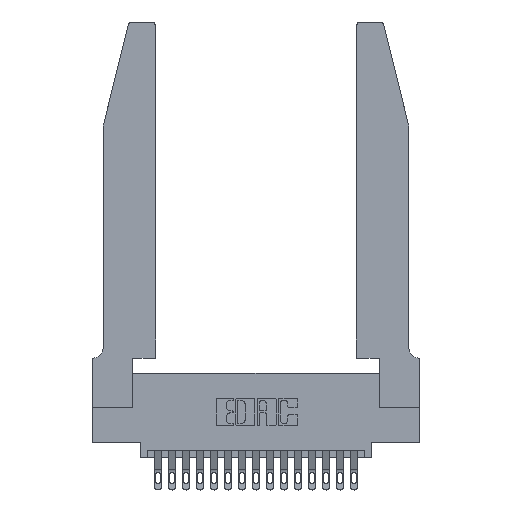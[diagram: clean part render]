
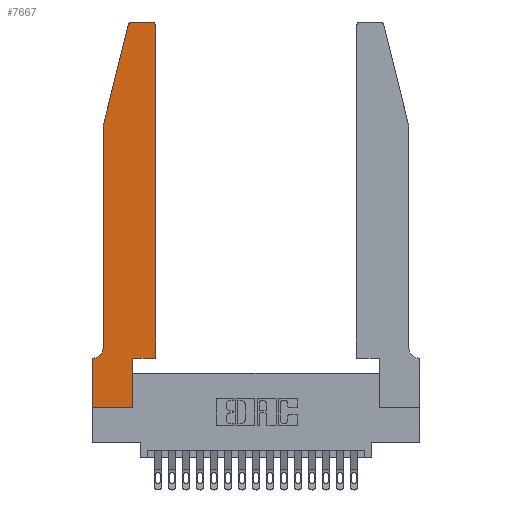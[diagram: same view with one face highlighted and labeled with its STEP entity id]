
A CAD part, top view. The second image highlights one B-rep face of the part: STEP entity #7667.
In plain terms, the highlighted planar face has unit normal (0, 0, 1).
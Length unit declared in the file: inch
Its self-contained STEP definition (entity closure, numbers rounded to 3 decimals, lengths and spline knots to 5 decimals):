
#40 = VERTEX_POINT ( 'NONE', #2530 ) ;
#57 = CARTESIAN_POINT ( 'NONE',  ( 0., 0., 0.37 ) ) ;
#232 = VERTEX_POINT ( 'NONE', #11182 ) ;
#585 = CARTESIAN_POINT ( 'NONE',  ( 0.2605, 2.75, 0.37 ) ) ;
#728 = VECTOR ( 'NONE', #1380, 39.37008 ) ;
#1380 = DIRECTION ( 'NONE',  ( 1., 0., 0. ) ) ;
#2530 = CARTESIAN_POINT ( 'NONE',  ( 0.25487, 2.72718, 0.37 ) ) ;
#2586 = VECTOR ( 'NONE', #4347, 39.37008 ) ;
#2841 = AXIS2_PLACEMENT_3D ( 'NONE', #10118, #5791, #13839 ) ;
#2979 = ORIENTED_EDGE ( 'NONE', *, *, #18411, .T. ) ;
#3191 = VERTEX_POINT ( 'NONE', #17429 ) ;
#3565 = CARTESIAN_POINT ( 'NONE',  ( 0., 0., 0.37 ) ) ;
#3614 = EDGE_CURVE ( 'NONE', #40, #8556, #8418, .T. ) ;
#3856 = AXIS2_PLACEMENT_3D ( 'NONE', #6709, #17944, #13166 ) ;
#3888 = EDGE_CURVE ( 'NONE', #16917, #5561, #12679, .T. ) ;
#4110 = ORIENTED_EDGE ( 'NONE', *, *, #10051, .T. ) ;
#4347 = DIRECTION ( 'NONE',  ( 0., -1., 0. ) ) ;
#4677 = CARTESIAN_POINT ( 'NONE',  ( 0.2865, 0., 0.37 ) ) ;
#4692 = CARTESIAN_POINT ( 'NONE',  ( 0., 0., 0.37 ) ) ;
#4755 = AXIS2_PLACEMENT_3D ( 'NONE', #7653, #12594, #9204 ) ;
#5081 = LINE ( 'NONE', #585, #10305 ) ;
#5183 = EDGE_CURVE ( 'NONE', #5561, #14321, #7615, .T. ) ;
#5474 = ORIENTED_EDGE ( 'NONE', *, *, #9919, .T. ) ;
#5485 = LINE ( 'NONE', #57, #728 ) ;
#5500 = ORIENTED_EDGE ( 'NONE', *, *, #6899, .T. ) ;
#5561 = VERTEX_POINT ( 'NONE', #11000 ) ;
#5791 = DIRECTION ( 'NONE',  ( 0., 0., 1. ) ) ;
#5873 = DIRECTION ( 'NONE',  ( 0., 0., 1. ) ) ;
#6017 = VECTOR ( 'NONE', #9428, 39.37008 ) ;
#6091 = LINE ( 'NONE', #9162, #2586 ) ;
#6281 = CIRCLE ( 'NONE', #3856, 0.03 ) ;
#6568 = EDGE_CURVE ( 'NONE', #8556, #16917, #6091, .T. ) ;
#6709 = CARTESIAN_POINT ( 'NONE',  ( 0.4205, 2.72, 0.37 ) ) ;
#6899 = EDGE_CURVE ( 'NONE', #232, #12903, #5081, .T. ) ;
#6917 = ORIENTED_EDGE ( 'NONE', *, *, #11841, .T. ) ;
#7072 = CARTESIAN_POINT ( 'NONE',  ( 0., 0.35, 0.37 ) ) ;
#7615 = LINE ( 'NONE', #15727, #12909 ) ;
#7653 = CARTESIAN_POINT ( 'NONE',  ( 0.0055, 0.42, 0.37 ) ) ;
#7667 = ADVANCED_FACE ( 'NONE', ( #14831 ), #9023, .T. ) ;
#7739 = DIRECTION ( 'NONE',  ( -1., 0., 0. ) ) ;
#7962 = EDGE_CURVE ( 'NONE', #3191, #232, #6281, .T. ) ;
#8030 = VERTEX_POINT ( 'NONE', #18083 ) ;
#8418 = LINE ( 'NONE', #9877, #16181 ) ;
#8556 = VERTEX_POINT ( 'NONE', #19950 ) ;
#8760 = ORIENTED_EDGE ( 'NONE', *, *, #9434, .T. ) ;
#8958 = CARTESIAN_POINT ( 'NONE',  ( 0.2865, 0.35, 0.37 ) ) ;
#9023 = PLANE ( 'NONE',  #11771 ) ;
#9162 = CARTESIAN_POINT ( 'NONE',  ( 0.0755, 2., 0.37 ) ) ;
#9168 = LINE ( 'NONE', #12380, #14961 ) ;
#9204 = DIRECTION ( 'NONE',  ( -1., 0., 0. ) ) ;
#9220 = DIRECTION ( 'NONE',  ( 1., 0., 0. ) ) ;
#9428 = DIRECTION ( 'NONE',  ( 0., -1., 0. ) ) ;
#9434 = EDGE_CURVE ( 'NONE', #8030, #3191, #11290, .T. ) ;
#9614 = CARTESIAN_POINT ( 'NONE',  ( 0.284, 2.75, 0.37 ) ) ;
#9857 = CARTESIAN_POINT ( 'NONE',  ( 0.2865, 0.35, 0.37 ) ) ;
#9877 = CARTESIAN_POINT ( 'NONE',  ( 0.0755, 2., 0.37 ) ) ;
#9919 = EDGE_CURVE ( 'NONE', #11551, #13581, #5485, .T. ) ;
#10051 = EDGE_CURVE ( 'NONE', #12903, #40, #12504, .T. ) ;
#10079 = DIRECTION ( 'NONE',  ( -0.239, -0.971, 0. ) ) ;
#10118 = CARTESIAN_POINT ( 'NONE',  ( 0.284, 2.72, 0.37 ) ) ;
#10142 = ORIENTED_EDGE ( 'NONE', *, *, #5183, .T. ) ;
#10295 = LINE ( 'NONE', #8958, #14060 ) ;
#10305 = VECTOR ( 'NONE', #15006, 39.37008 ) ;
#10430 = CARTESIAN_POINT ( 'NONE',  ( 0.4505, 0.35, 0.37 ) ) ;
#10916 = ORIENTED_EDGE ( 'NONE', *, *, #13179, .T. ) ;
#11000 = CARTESIAN_POINT ( 'NONE',  ( 0.0055, 0.35, 0.37 ) ) ;
#11182 = CARTESIAN_POINT ( 'NONE',  ( 0.4205, 2.75, 0.37 ) ) ;
#11290 = LINE ( 'NONE', #10430, #20212 ) ;
#11551 = VERTEX_POINT ( 'NONE', #3565 ) ;
#11652 = ORIENTED_EDGE ( 'NONE', *, *, #7962, .T. ) ;
#11771 = AXIS2_PLACEMENT_3D ( 'NONE', #18684, #5873, #20140 ) ;
#11841 = EDGE_CURVE ( 'NONE', #12798, #8030, #9168, .T. ) ;
#12380 = CARTESIAN_POINT ( 'NONE',  ( 0.4505, 0.35, 0.37 ) ) ;
#12504 = CIRCLE ( 'NONE', #2841, 0.03 ) ;
#12594 = DIRECTION ( 'NONE',  ( 0., 0., -1. ) ) ;
#12679 = CIRCLE ( 'NONE', #4755, 0.07 ) ;
#12798 = VERTEX_POINT ( 'NONE', #9857 ) ;
#12903 = VERTEX_POINT ( 'NONE', #9614 ) ;
#12909 = VECTOR ( 'NONE', #7739, 39.37008 ) ;
#13166 = DIRECTION ( 'NONE',  ( 1., 0., 0. ) ) ;
#13179 = EDGE_CURVE ( 'NONE', #13581, #12798, #10295, .T. ) ;
#13581 = VERTEX_POINT ( 'NONE', #4677 ) ;
#13839 = DIRECTION ( 'NONE',  ( 1., 0., 0. ) ) ;
#14060 = VECTOR ( 'NONE', #20078, 39.37008 ) ;
#14321 = VERTEX_POINT ( 'NONE', #7072 ) ;
#14358 = CARTESIAN_POINT ( 'NONE',  ( 0.0755, 0.42, 0.37 ) ) ;
#14831 = FACE_OUTER_BOUND ( 'NONE', #18434, .T. ) ;
#14961 = VECTOR ( 'NONE', #9220, 39.37008 ) ;
#15006 = DIRECTION ( 'NONE',  ( -1., 0., 0. ) ) ;
#15149 = DIRECTION ( 'NONE',  ( 0., 1., 0. ) ) ;
#15727 = CARTESIAN_POINT ( 'NONE',  ( 0.0755, 0.35, 0.37 ) ) ;
#16181 = VECTOR ( 'NONE', #10079, 39.37008 ) ;
#16917 = VERTEX_POINT ( 'NONE', #14358 ) ;
#17429 = CARTESIAN_POINT ( 'NONE',  ( 0.4505, 2.72, 0.37 ) ) ;
#17944 = DIRECTION ( 'NONE',  ( 0., 0., 1. ) ) ;
#18083 = CARTESIAN_POINT ( 'NONE',  ( 0.4505, 0.35, 0.37 ) ) ;
#18205 = ORIENTED_EDGE ( 'NONE', *, *, #3888, .T. ) ;
#18411 = EDGE_CURVE ( 'NONE', #14321, #11551, #19959, .T. ) ;
#18434 = EDGE_LOOP ( 'NONE', ( #5500, #4110, #20131, #20263, #18205, #10142, #2979, #5474, #10916, #6917, #8760, #11652 ) ) ;
#18684 = CARTESIAN_POINT ( 'NONE',  ( 0., 0.35, 0.37 ) ) ;
#19950 = CARTESIAN_POINT ( 'NONE',  ( 0.0755, 2., 0.37 ) ) ;
#19959 = LINE ( 'NONE', #4692, #6017 ) ;
#20078 = DIRECTION ( 'NONE',  ( 0., 1., 0. ) ) ;
#20131 = ORIENTED_EDGE ( 'NONE', *, *, #3614, .T. ) ;
#20140 = DIRECTION ( 'NONE',  ( 1., 0., 0. ) ) ;
#20212 = VECTOR ( 'NONE', #15149, 39.37008 ) ;
#20263 = ORIENTED_EDGE ( 'NONE', *, *, #6568, .T. ) ;
